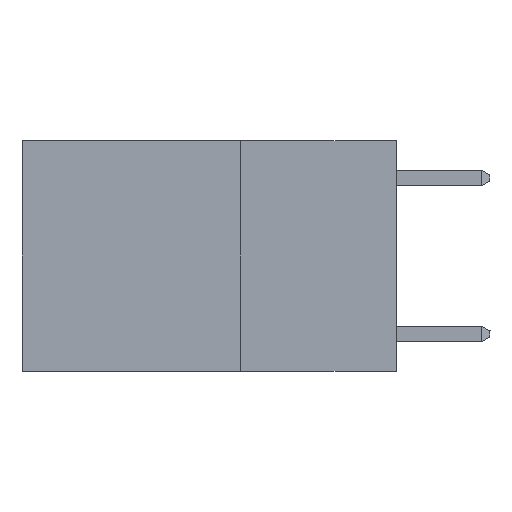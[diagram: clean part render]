
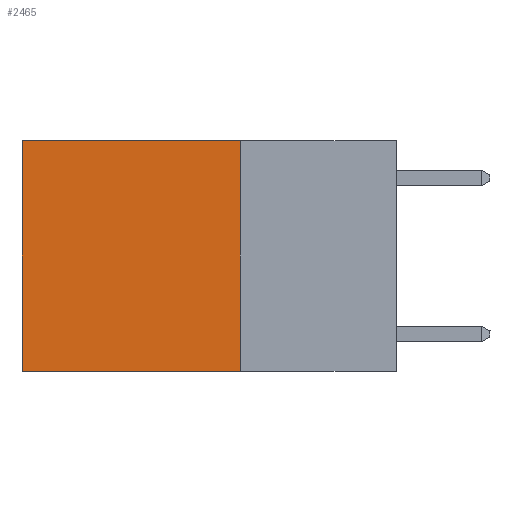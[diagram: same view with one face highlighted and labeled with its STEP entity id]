
A CAD part, left-side view. The second image highlights one B-rep face of the part: STEP entity #2465.
In plain terms, the highlighted planar face has unit normal (-1, 0, 0).
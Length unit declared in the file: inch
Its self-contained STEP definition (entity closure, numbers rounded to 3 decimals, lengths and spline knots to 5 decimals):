
#82 = EDGE_CURVE ( 'NONE', #577, #27308, #22400, .T. ) ;
#577 = VERTEX_POINT ( 'NONE', #18481 ) ;
#2465 = ADVANCED_FACE ( 'NONE', ( #7922 ), #17827, .F. ) ;
#6184 = LINE ( 'NONE', #15887, #25069 ) ;
#6208 = VECTOR ( 'NONE', #20326, 39.37008 ) ;
#6628 = ORIENTED_EDGE ( 'NONE', *, *, #10901, .T. ) ;
#7922 = FACE_OUTER_BOUND ( 'NONE', #25924, .T. ) ;
#8204 = CARTESIAN_POINT ( 'NONE',  ( 0.2625, 0.25, 0. ) ) ;
#10177 = VECTOR ( 'NONE', #22439, 39.37008 ) ;
#10901 = EDGE_CURVE ( 'NONE', #14714, #27308, #12176, .T. ) ;
#10977 = EDGE_CURVE ( 'NONE', #11317, #577, #6184, .T. ) ;
#11317 = VERTEX_POINT ( 'NONE', #8204 ) ;
#12176 = LINE ( 'NONE', #16199, #6208 ) ;
#12670 = AXIS2_PLACEMENT_3D ( 'NONE', #22336, #15417, #24421 ) ;
#12976 = CARTESIAN_POINT ( 'NONE',  ( 0.2625, 0.6, 0. ) ) ;
#14377 = LINE ( 'NONE', #28156, #21746 ) ;
#14714 = VERTEX_POINT ( 'NONE', #12976 ) ;
#15417 = DIRECTION ( 'NONE',  ( 1., 0., 0. ) ) ;
#15831 = ORIENTED_EDGE ( 'NONE', *, *, #17614, .T. ) ;
#15887 = CARTESIAN_POINT ( 'NONE',  ( 0.2625, 0.25, 0. ) ) ;
#15999 = CARTESIAN_POINT ( 'NONE',  ( 0.2625, 0.25, -0.37 ) ) ;
#16199 = CARTESIAN_POINT ( 'NONE',  ( 0.2625, 0.6, 0. ) ) ;
#16928 = DIRECTION ( 'NONE',  ( 0., 1., 0. ) ) ;
#17614 = EDGE_CURVE ( 'NONE', #11317, #14714, #14377, .T. ) ;
#17706 = CARTESIAN_POINT ( 'NONE',  ( 0.2625, 0.6, -0.37 ) ) ;
#17827 = PLANE ( 'NONE',  #12670 ) ;
#18481 = CARTESIAN_POINT ( 'NONE',  ( 0.2625, 0.25, -0.37 ) ) ;
#20215 = DIRECTION ( 'NONE',  ( 0., 0., -1. ) ) ;
#20326 = DIRECTION ( 'NONE',  ( 0., 0., -1. ) ) ;
#21746 = VECTOR ( 'NONE', #16928, 39.37008 ) ;
#22044 = ORIENTED_EDGE ( 'NONE', *, *, #82, .F. ) ;
#22336 = CARTESIAN_POINT ( 'NONE',  ( 0.2625, 0.25, 0. ) ) ;
#22400 = LINE ( 'NONE', #15999, #10177 ) ;
#22439 = DIRECTION ( 'NONE',  ( 0., 1., 0. ) ) ;
#24421 = DIRECTION ( 'NONE',  ( 0., 0., -1. ) ) ;
#25069 = VECTOR ( 'NONE', #20215, 39.37008 ) ;
#25924 = EDGE_LOOP ( 'NONE', ( #6628, #22044, #27060, #15831 ) ) ;
#27060 = ORIENTED_EDGE ( 'NONE', *, *, #10977, .F. ) ;
#27308 = VERTEX_POINT ( 'NONE', #17706 ) ;
#28156 = CARTESIAN_POINT ( 'NONE',  ( 0.2625, 0.25, 0. ) ) ;
